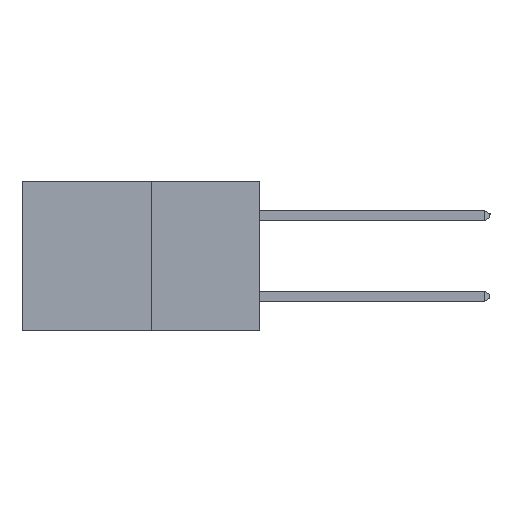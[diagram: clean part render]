
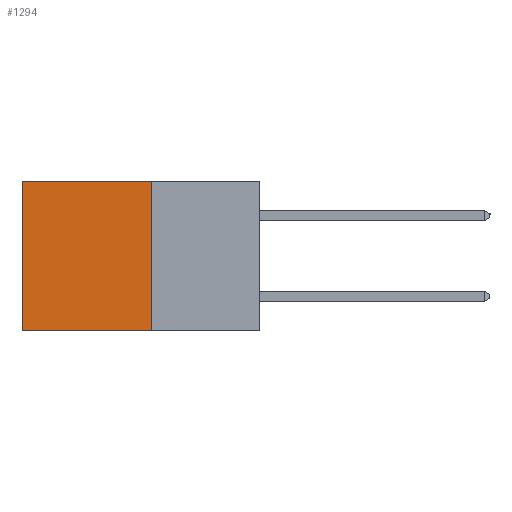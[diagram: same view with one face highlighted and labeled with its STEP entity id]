
A CAD part, left-side view. The second image highlights one B-rep face of the part: STEP entity #1294.
In plain terms, the highlighted planar face has unit normal (-1, 0, 0).
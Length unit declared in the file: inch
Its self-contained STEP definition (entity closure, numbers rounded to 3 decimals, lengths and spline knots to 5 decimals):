
#375 = ORIENTED_EDGE ( 'NONE', *, *, #3687, .F. ) ;
#471 = EDGE_CURVE ( 'NONE', #7136, #3027, #5617, .T. ) ;
#640 = ORIENTED_EDGE ( 'NONE', *, *, #810, .F. ) ;
#810 = EDGE_CURVE ( 'NONE', #5700, #7472, #8949, .T. ) ;
#1282 = DIRECTION ( 'NONE',  ( 0., 1., 0. ) ) ;
#1294 = ADVANCED_FACE ( 'NONE', ( #1533 ), #2536, .F. ) ;
#1533 = FACE_OUTER_BOUND ( 'NONE', #6834, .T. ) ;
#1728 = CARTESIAN_POINT ( 'NONE',  ( 0.277, 0.27, -0.37 ) ) ;
#2282 = CARTESIAN_POINT ( 'NONE',  ( 0.277, 0.59, -0.37 ) ) ;
#2405 = VECTOR ( 'NONE', #3232, 39.37008 ) ;
#2536 = PLANE ( 'NONE',  #3179 ) ;
#3027 = VERTEX_POINT ( 'NONE', #5384 ) ;
#3137 = CARTESIAN_POINT ( 'NONE',  ( 0.277, 0.27, -0.37 ) ) ;
#3179 = AXIS2_PLACEMENT_3D ( 'NONE', #3209, #6561, #3750 ) ;
#3209 = CARTESIAN_POINT ( 'NONE',  ( 0.277, 0.27, -0.37 ) ) ;
#3232 = DIRECTION ( 'NONE',  ( 0., 0., -1. ) ) ;
#3687 = EDGE_CURVE ( 'NONE', #7136, #5700, #4304, .T. ) ;
#3750 = DIRECTION ( 'NONE',  ( 0., 0., -1. ) ) ;
#3942 = VECTOR ( 'NONE', #7850, 39.37008 ) ;
#4056 = VECTOR ( 'NONE', #1282, 39.37008 ) ;
#4304 = LINE ( 'NONE', #1728, #2405 ) ;
#5092 = DIRECTION ( 'NONE',  ( 0., 0., -1. ) ) ;
#5105 = EDGE_CURVE ( 'NONE', #3027, #7472, #7412, .T. ) ;
#5384 = CARTESIAN_POINT ( 'NONE',  ( 0.277, 0.59, 0. ) ) ;
#5617 = LINE ( 'NONE', #5626, #4056 ) ;
#5620 = VECTOR ( 'NONE', #5092, 39.37008 ) ;
#5626 = CARTESIAN_POINT ( 'NONE',  ( 0.277, 0.27, 0. ) ) ;
#5700 = VERTEX_POINT ( 'NONE', #8704 ) ;
#5789 = ORIENTED_EDGE ( 'NONE', *, *, #471, .T. ) ;
#6383 = ORIENTED_EDGE ( 'NONE', *, *, #5105, .T. ) ;
#6561 = DIRECTION ( 'NONE',  ( 1., 0., 0. ) ) ;
#6834 = EDGE_LOOP ( 'NONE', ( #6383, #640, #375, #5789 ) ) ;
#7136 = VERTEX_POINT ( 'NONE', #8827 ) ;
#7412 = LINE ( 'NONE', #8370, #5620 ) ;
#7472 = VERTEX_POINT ( 'NONE', #2282 ) ;
#7850 = DIRECTION ( 'NONE',  ( 0., 1., 0. ) ) ;
#8370 = CARTESIAN_POINT ( 'NONE',  ( 0.277, 0.59, -0.37 ) ) ;
#8704 = CARTESIAN_POINT ( 'NONE',  ( 0.277, 0.27, -0.37 ) ) ;
#8827 = CARTESIAN_POINT ( 'NONE',  ( 0.277, 0.27, 0. ) ) ;
#8949 = LINE ( 'NONE', #3137, #3942 ) ;
